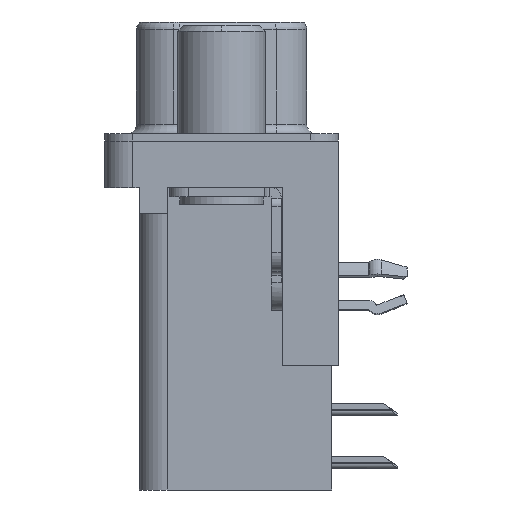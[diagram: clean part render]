
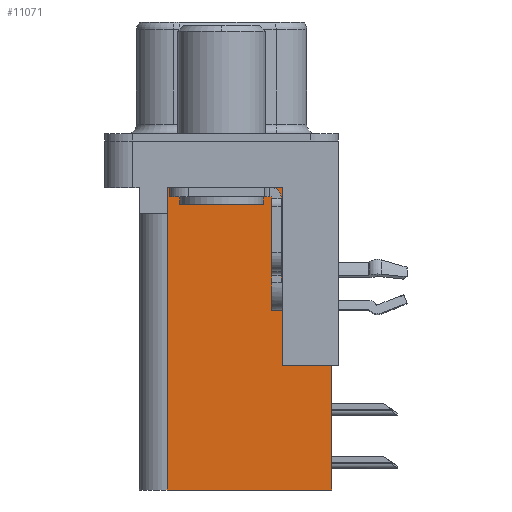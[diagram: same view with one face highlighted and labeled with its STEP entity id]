
A CAD part, left-side view. The second image highlights one B-rep face of the part: STEP entity #11071.
In plain terms, the highlighted planar face has unit normal (-1, 0, 0).
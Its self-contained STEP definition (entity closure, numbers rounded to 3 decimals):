
#328 = VERTEX_POINT ( 'NONE', #20642 ) ;
#638 = VERTEX_POINT ( 'NONE', #1202 ) ;
#647 = VECTOR ( 'NONE', #14335, 1000. ) ;
#963 = CARTESIAN_POINT ( 'NONE',  ( 3.7, 2.925, -18.76 ) ) ;
#1202 = CARTESIAN_POINT ( 'NONE',  ( 3.7, 2.895, -3.9 ) ) ;
#1222 = EDGE_CURVE ( 'NONE', #638, #328, #8277, .T. ) ;
#1276 = CARTESIAN_POINT ( 'NONE',  ( 3.7, -6.295, -12.05 ) ) ;
#1454 = EDGE_CURVE ( 'NONE', #14402, #18213, #3576, .T. ) ;
#1719 = CARTESIAN_POINT ( 'NONE',  ( 3.7, 2.925, -18.76 ) ) ;
#2709 = AXIS2_PLACEMENT_3D ( 'NONE', #16333, #22149, #10633 ) ;
#3081 = CARTESIAN_POINT ( 'NONE',  ( 3.7, -3.295, -2.5 ) ) ;
#3576 = LINE ( 'NONE', #5835, #18135 ) ;
#4000 = ORIENTED_EDGE ( 'NONE', *, *, #13020, .T. ) ;
#4034 = DIRECTION ( 'NONE',  ( 0., 1., 0. ) ) ;
#4468 = VECTOR ( 'NONE', #23324, 1000. ) ;
#4798 = CARTESIAN_POINT ( 'NONE',  ( 3.7, -3.295, -2.5 ) ) ;
#4857 = LINE ( 'NONE', #3081, #19463 ) ;
#5011 = EDGE_CURVE ( 'NONE', #9044, #638, #15718, .T. ) ;
#5671 = ORIENTED_EDGE ( 'NONE', *, *, #5011, .T. ) ;
#5732 = LINE ( 'NONE', #963, #15236 ) ;
#5835 = CARTESIAN_POINT ( 'NONE',  ( 3.7, -3.295, -18.76 ) ) ;
#6653 = LINE ( 'NONE', #1276, #16766 ) ;
#7006 = VECTOR ( 'NONE', #10505, 1000. ) ;
#7019 = FACE_OUTER_BOUND ( 'NONE', #12419, .T. ) ;
#8100 = VERTEX_POINT ( 'NONE', #10843 ) ;
#8277 = LINE ( 'NONE', #9919, #22977 ) ;
#8617 = EDGE_CURVE ( 'NONE', #18213, #9044, #4857, .T. ) ;
#8963 = CARTESIAN_POINT ( 'NONE',  ( 3.7, 2.895, -3.9 ) ) ;
#9044 = VERTEX_POINT ( 'NONE', #9478 ) ;
#9478 = CARTESIAN_POINT ( 'NONE',  ( 3.7, 2.895, -2.5 ) ) ;
#9759 = ORIENTED_EDGE ( 'NONE', *, *, #1222, .T. ) ;
#9919 = CARTESIAN_POINT ( 'NONE',  ( 3.7, 0., -3.9 ) ) ;
#10505 = DIRECTION ( 'NONE',  ( 0., 0., -1. ) ) ;
#10633 = DIRECTION ( 'NONE',  ( 0., 1., 0. ) ) ;
#10843 = CARTESIAN_POINT ( 'NONE',  ( 3.7, -5.925, -12.05 ) ) ;
#11071 = ADVANCED_FACE ( 'NONE', ( #7019 ), #20185, .F. ) ;
#11391 = VERTEX_POINT ( 'NONE', #17171 ) ;
#12392 = CARTESIAN_POINT ( 'NONE',  ( 3.7, -5.925, -2. ) ) ;
#12419 = EDGE_LOOP ( 'NONE', ( #13173, #5671, #9759, #23498, #22709, #12846, #4000, #14455 ) ) ;
#12846 = ORIENTED_EDGE ( 'NONE', *, *, #18614, .F. ) ;
#13020 = EDGE_CURVE ( 'NONE', #8100, #14402, #6653, .T. ) ;
#13173 = ORIENTED_EDGE ( 'NONE', *, *, #8617, .T. ) ;
#14335 = DIRECTION ( 'NONE',  ( 0., 0., -1. ) ) ;
#14402 = VERTEX_POINT ( 'NONE', #21248 ) ;
#14455 = ORIENTED_EDGE ( 'NONE', *, *, #1454, .T. ) ;
#14611 = EDGE_CURVE ( 'NONE', #16253, #328, #5732, .T. ) ;
#15236 = VECTOR ( 'NONE', #16079, 1000. ) ;
#15718 = LINE ( 'NONE', #8963, #647 ) ;
#16079 = DIRECTION ( 'NONE',  ( 0., 0., 1. ) ) ;
#16253 = VERTEX_POINT ( 'NONE', #1719 ) ;
#16333 = CARTESIAN_POINT ( 'NONE',  ( 3.7, -3.295, -18.76 ) ) ;
#16766 = VECTOR ( 'NONE', #20257, 1000. ) ;
#17147 = LINE ( 'NONE', #12392, #7006 ) ;
#17171 = CARTESIAN_POINT ( 'NONE',  ( 3.7, -5.925, -18.76 ) ) ;
#18135 = VECTOR ( 'NONE', #23022, 1000. ) ;
#18213 = VERTEX_POINT ( 'NONE', #4798 ) ;
#18614 = EDGE_CURVE ( 'NONE', #8100, #11391, #17147, .T. ) ;
#19463 = VECTOR ( 'NONE', #20114, 1000. ) ;
#20114 = DIRECTION ( 'NONE',  ( 0., 1., 0. ) ) ;
#20185 = PLANE ( 'NONE',  #2709 ) ;
#20257 = DIRECTION ( 'NONE',  ( 0., 1., 0. ) ) ;
#20642 = CARTESIAN_POINT ( 'NONE',  ( 3.7, 2.925, -3.9 ) ) ;
#21248 = CARTESIAN_POINT ( 'NONE',  ( 3.7, -3.295, -12.05 ) ) ;
#21407 = CARTESIAN_POINT ( 'NONE',  ( 3.7, -3.295, -18.76 ) ) ;
#22149 = DIRECTION ( 'NONE',  ( 1., 0., 0. ) ) ;
#22709 = ORIENTED_EDGE ( 'NONE', *, *, #22969, .F. ) ;
#22969 = EDGE_CURVE ( 'NONE', #11391, #16253, #24152, .T. ) ;
#22977 = VECTOR ( 'NONE', #4034, 1000. ) ;
#23022 = DIRECTION ( 'NONE',  ( 0., 0., 1. ) ) ;
#23324 = DIRECTION ( 'NONE',  ( 0., 1., 0. ) ) ;
#23498 = ORIENTED_EDGE ( 'NONE', *, *, #14611, .F. ) ;
#24152 = LINE ( 'NONE', #21407, #4468 ) ;
